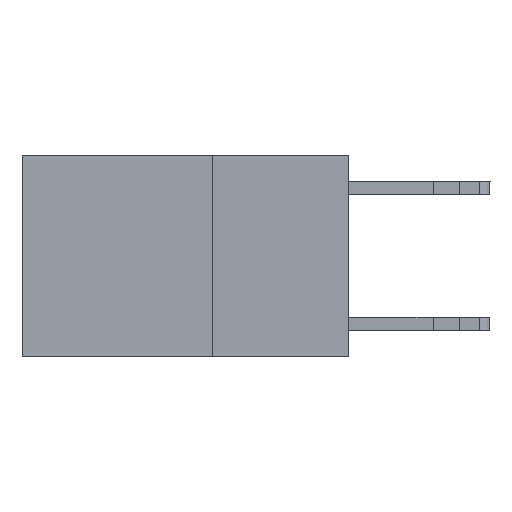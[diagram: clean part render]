
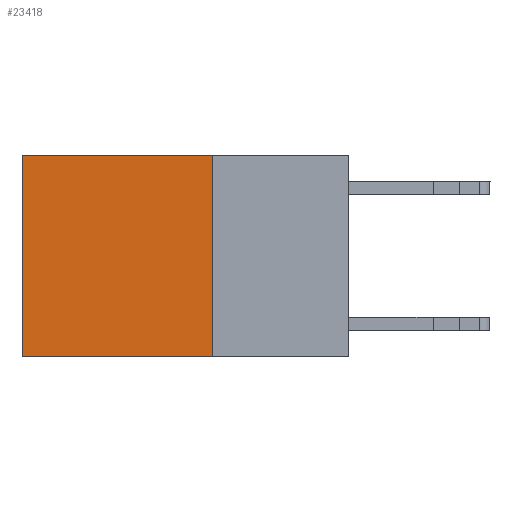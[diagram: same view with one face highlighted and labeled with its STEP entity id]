
A CAD part, left-side view. The second image highlights one B-rep face of the part: STEP entity #23418.
In plain terms, the highlighted planar face has unit normal (-1, 0, 0).
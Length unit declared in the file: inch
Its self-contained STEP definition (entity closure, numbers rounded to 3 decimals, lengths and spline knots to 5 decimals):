
#258 = ORIENTED_EDGE ( 'NONE', *, *, #2093, .F. ) ;
#308 = LINE ( 'NONE', #4349, #20108 ) ;
#2052 = DIRECTION ( 'NONE',  ( 0., 0., -1. ) ) ;
#2093 = EDGE_CURVE ( 'NONE', #9580, #16846, #22926, .T. ) ;
#2155 = CARTESIAN_POINT ( 'NONE',  ( 0.2625, 0.6, -0.37 ) ) ;
#4063 = VERTEX_POINT ( 'NONE', #2155 ) ;
#4349 = CARTESIAN_POINT ( 'NONE',  ( 0.2625, 0.25, 0. ) ) ;
#4629 = VECTOR ( 'NONE', #20380, 39.37008 ) ;
#5118 = CARTESIAN_POINT ( 'NONE',  ( 0.2625, 0.25, 0. ) ) ;
#6446 = CARTESIAN_POINT ( 'NONE',  ( 0.2625, 0.25, 0. ) ) ;
#8048 = CARTESIAN_POINT ( 'NONE',  ( 0.2625, 0.6, 0. ) ) ;
#8749 = FACE_OUTER_BOUND ( 'NONE', #8805, .T. ) ;
#8805 = EDGE_LOOP ( 'NONE', ( #18897, #12711, #258, #11332 ) ) ;
#9446 = CARTESIAN_POINT ( 'NONE',  ( 0.2625, 0.25, 0. ) ) ;
#9580 = VERTEX_POINT ( 'NONE', #6446 ) ;
#10495 = CARTESIAN_POINT ( 'NONE',  ( 0.2625, 0.25, -0.37 ) ) ;
#10730 = LINE ( 'NONE', #16346, #15384 ) ;
#11332 = ORIENTED_EDGE ( 'NONE', *, *, #23632, .T. ) ;
#12711 = ORIENTED_EDGE ( 'NONE', *, *, #21290, .F. ) ;
#13544 = VERTEX_POINT ( 'NONE', #8048 ) ;
#15384 = VECTOR ( 'NONE', #23729, 39.37008 ) ;
#16346 = CARTESIAN_POINT ( 'NONE',  ( 0.2625, 0.6, 0. ) ) ;
#16846 = VERTEX_POINT ( 'NONE', #10495 ) ;
#18169 = AXIS2_PLACEMENT_3D ( 'NONE', #5118, #20327, #22712 ) ;
#18379 = LINE ( 'NONE', #18498, #4629 ) ;
#18498 = CARTESIAN_POINT ( 'NONE',  ( 0.2625, 0.25, -0.37 ) ) ;
#18897 = ORIENTED_EDGE ( 'NONE', *, *, #19693, .T. ) ;
#19481 = VECTOR ( 'NONE', #2052, 39.37008 ) ;
#19671 = DIRECTION ( 'NONE',  ( 0., 1., 0. ) ) ;
#19693 = EDGE_CURVE ( 'NONE', #13544, #4063, #10730, .T. ) ;
#20108 = VECTOR ( 'NONE', #19671, 39.37008 ) ;
#20327 = DIRECTION ( 'NONE',  ( 1., 0., 0. ) ) ;
#20380 = DIRECTION ( 'NONE',  ( 0., 1., 0. ) ) ;
#21290 = EDGE_CURVE ( 'NONE', #16846, #4063, #18379, .T. ) ;
#22712 = DIRECTION ( 'NONE',  ( 0., 0., -1. ) ) ;
#22926 = LINE ( 'NONE', #9446, #19481 ) ;
#23418 = ADVANCED_FACE ( 'NONE', ( #8749 ), #23956, .F. ) ;
#23632 = EDGE_CURVE ( 'NONE', #9580, #13544, #308, .T. ) ;
#23729 = DIRECTION ( 'NONE',  ( 0., 0., -1. ) ) ;
#23956 = PLANE ( 'NONE',  #18169 ) ;
